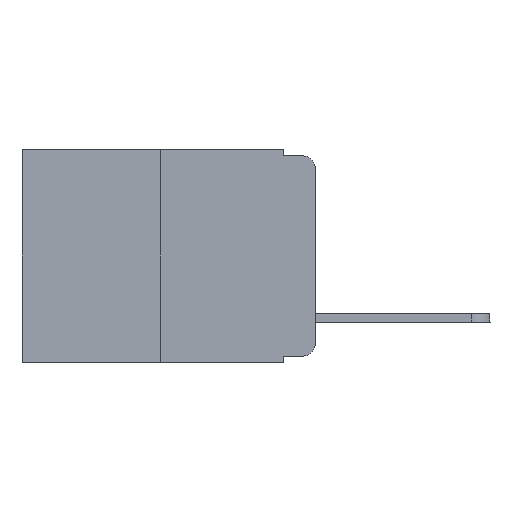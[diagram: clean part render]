
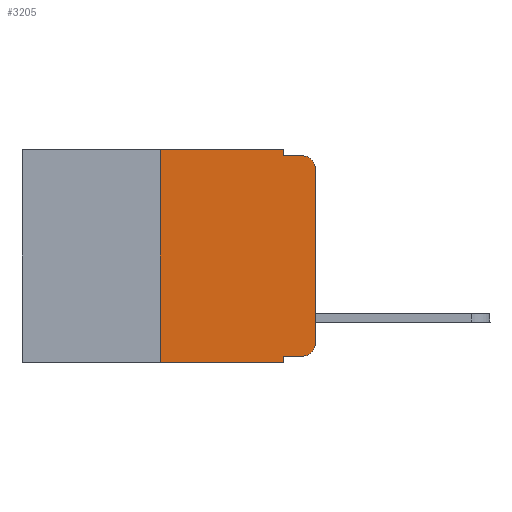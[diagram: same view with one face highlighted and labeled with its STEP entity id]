
A CAD part, left-side view. The second image highlights one B-rep face of the part: STEP entity #3205.
In plain terms, the highlighted planar face has unit normal (-1, 0, 0).
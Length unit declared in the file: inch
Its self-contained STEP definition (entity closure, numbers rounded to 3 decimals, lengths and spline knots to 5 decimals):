
#17 = EDGE_CURVE ( 'NONE', #14859, #660, #18281, .T. ) ;
#322 = ORIENTED_EDGE ( 'NONE', *, *, #17, .F. ) ;
#340 = CARTESIAN_POINT ( 'NONE',  ( 0., 0.25, -0.343 ) ) ;
#506 = LINE ( 'NONE', #2362, #17073 ) ;
#578 = DIRECTION ( 'NONE',  ( 0., -1., 0. ) ) ;
#582 = ORIENTED_EDGE ( 'NONE', *, *, #11948, .F. ) ;
#660 = VERTEX_POINT ( 'NONE', #14155 ) ;
#1034 = CARTESIAN_POINT ( 'NONE',  ( 0., 0.02, -0.01 ) ) ;
#1178 = EDGE_CURVE ( 'NONE', #11960, #11316, #10306, .T. ) ;
#1260 = ORIENTED_EDGE ( 'NONE', *, *, #17688, .T. ) ;
#2116 = DIRECTION ( 'NONE',  ( 1., 0., 0. ) ) ;
#2301 = EDGE_CURVE ( 'NONE', #11316, #20093, #506, .T. ) ;
#2362 = CARTESIAN_POINT ( 'NONE',  ( 0., 0., 0. ) ) ;
#2386 = FACE_OUTER_BOUND ( 'NONE', #9020, .T. ) ;
#2668 = VECTOR ( 'NONE', #20241, 39.37008 ) ;
#2825 = CARTESIAN_POINT ( 'NONE',  ( 0., 0.25, 0. ) ) ;
#2946 = DIRECTION ( 'NONE',  ( 0., 0., -1. ) ) ;
#3034 = EDGE_CURVE ( 'NONE', #10674, #17400, #6200, .T. ) ;
#3205 = ADVANCED_FACE ( 'NONE', ( #2386 ), #20710, .F. ) ;
#3725 = DIRECTION ( 'NONE',  ( 0., 0., -1. ) ) ;
#4147 = AXIS2_PLACEMENT_3D ( 'NONE', #19422, #17763, #3725 ) ;
#4950 = ORIENTED_EDGE ( 'NONE', *, *, #15814, .F. ) ;
#5077 = VERTEX_POINT ( 'NONE', #18935 ) ;
#5681 = ORIENTED_EDGE ( 'NONE', *, *, #1178, .T. ) ;
#6200 = LINE ( 'NONE', #21656, #2668 ) ;
#6660 = VECTOR ( 'NONE', #6984, 39.37008 ) ;
#6690 = LINE ( 'NONE', #21088, #6660 ) ;
#6984 = DIRECTION ( 'NONE',  ( 0., 0., -1. ) ) ;
#7329 = VERTEX_POINT ( 'NONE', #10508 ) ;
#7890 = ORIENTED_EDGE ( 'NONE', *, *, #18589, .F. ) ;
#8533 = DIRECTION ( 'NONE',  ( 0., -1., 0. ) ) ;
#8685 = VECTOR ( 'NONE', #20239, 39.37008 ) ;
#8747 = CARTESIAN_POINT ( 'NONE',  ( 0., 0.051, -0.333 ) ) ;
#9020 = EDGE_LOOP ( 'NONE', ( #18112, #13419, #9094, #7890, #322, #4950, #10037, #582, #1260, #5681 ) ) ;
#9036 = VECTOR ( 'NONE', #578, 39.37008 ) ;
#9094 = ORIENTED_EDGE ( 'NONE', *, *, #3034, .F. ) ;
#9184 = CARTESIAN_POINT ( 'NONE',  ( 0., 0.02, -0.333 ) ) ;
#9781 = CARTESIAN_POINT ( 'NONE',  ( 0., 0.051, 0. ) ) ;
#10037 = ORIENTED_EDGE ( 'NONE', *, *, #18714, .T. ) ;
#10290 = VECTOR ( 'NONE', #21958, 39.37008 ) ;
#10306 = CIRCLE ( 'NONE', #4147, 0.02 ) ;
#10364 = VERTEX_POINT ( 'NONE', #340 ) ;
#10508 = CARTESIAN_POINT ( 'NONE',  ( 0., 0.051, -0.333 ) ) ;
#10585 = CARTESIAN_POINT ( 'NONE',  ( 0., 0.051, -0.01 ) ) ;
#10674 = VERTEX_POINT ( 'NONE', #10585 ) ;
#11163 = CARTESIAN_POINT ( 'NONE',  ( 0., 0.473, 0. ) ) ;
#11316 = VERTEX_POINT ( 'NONE', #18256 ) ;
#11352 = LINE ( 'NONE', #20460, #17628 ) ;
#11813 = AXIS2_PLACEMENT_3D ( 'NONE', #13324, #20383, #2946 ) ;
#11866 = DIRECTION ( 'NONE',  ( 0., -1., 0. ) ) ;
#11948 = EDGE_CURVE ( 'NONE', #7329, #5077, #6690, .T. ) ;
#11960 = VERTEX_POINT ( 'NONE', #9184 ) ;
#13283 = LINE ( 'NONE', #9781, #8685 ) ;
#13324 = CARTESIAN_POINT ( 'NONE',  ( 0., 0.02, -0.03 ) ) ;
#13419 = ORIENTED_EDGE ( 'NONE', *, *, #16821, .T. ) ;
#14155 = CARTESIAN_POINT ( 'NONE',  ( 0., 0.051, 0. ) ) ;
#14859 = VERTEX_POINT ( 'NONE', #16125 ) ;
#14916 = LINE ( 'NONE', #2825, #10290 ) ;
#15661 = LINE ( 'NONE', #8747, #21363 ) ;
#15814 = EDGE_CURVE ( 'NONE', #10364, #14859, #14916, .T. ) ;
#16125 = CARTESIAN_POINT ( 'NONE',  ( 0., 0.25, 0. ) ) ;
#16821 = EDGE_CURVE ( 'NONE', #20093, #17400, #18128, .T. ) ;
#17073 = VECTOR ( 'NONE', #20936, 39.37008 ) ;
#17400 = VERTEX_POINT ( 'NONE', #1034 ) ;
#17628 = VECTOR ( 'NONE', #11866, 39.37008 ) ;
#17688 = EDGE_CURVE ( 'NONE', #7329, #11960, #15661, .T. ) ;
#17749 = DIRECTION ( 'NONE',  ( 0., 0., -1. ) ) ;
#17763 = DIRECTION ( 'NONE',  ( -1., 0., 0. ) ) ;
#18112 = ORIENTED_EDGE ( 'NONE', *, *, #2301, .T. ) ;
#18128 = CIRCLE ( 'NONE', #11813, 0.02 ) ;
#18256 = CARTESIAN_POINT ( 'NONE',  ( 0., 0., -0.313 ) ) ;
#18281 = LINE ( 'NONE', #11163, #9036 ) ;
#18589 = EDGE_CURVE ( 'NONE', #660, #10674, #13283, .T. ) ;
#18714 = EDGE_CURVE ( 'NONE', #10364, #5077, #11352, .T. ) ;
#18935 = CARTESIAN_POINT ( 'NONE',  ( 0., 0.051, -0.343 ) ) ;
#19422 = CARTESIAN_POINT ( 'NONE',  ( 0., 0.02, -0.313 ) ) ;
#20093 = VERTEX_POINT ( 'NONE', #20632 ) ;
#20239 = DIRECTION ( 'NONE',  ( 0., 0., -1. ) ) ;
#20241 = DIRECTION ( 'NONE',  ( 0., -1., 0. ) ) ;
#20383 = DIRECTION ( 'NONE',  ( -1., 0., 0. ) ) ;
#20460 = CARTESIAN_POINT ( 'NONE',  ( 0., 0.473, -0.343 ) ) ;
#20632 = CARTESIAN_POINT ( 'NONE',  ( 0., 0., -0.03 ) ) ;
#20710 = PLANE ( 'NONE',  #21170 ) ;
#20936 = DIRECTION ( 'NONE',  ( 0., 0., 1. ) ) ;
#21088 = CARTESIAN_POINT ( 'NONE',  ( 0., 0.051, 0. ) ) ;
#21158 = CARTESIAN_POINT ( 'NONE',  ( 0., 0.473, 0. ) ) ;
#21170 = AXIS2_PLACEMENT_3D ( 'NONE', #21158, #2116, #17749 ) ;
#21363 = VECTOR ( 'NONE', #8533, 39.37008 ) ;
#21656 = CARTESIAN_POINT ( 'NONE',  ( 0., 0.051, -0.01 ) ) ;
#21958 = DIRECTION ( 'NONE',  ( 0., 0., 1. ) ) ;
